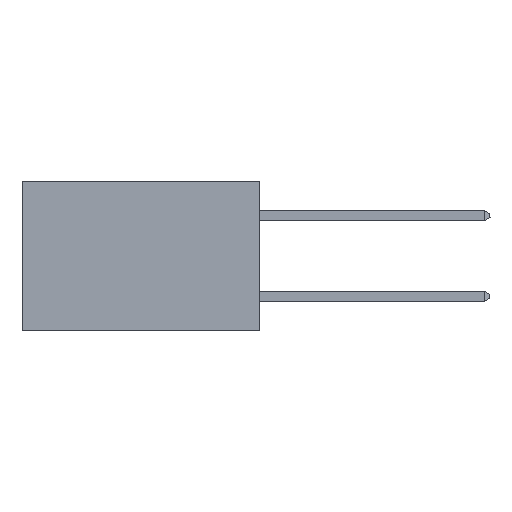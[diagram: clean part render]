
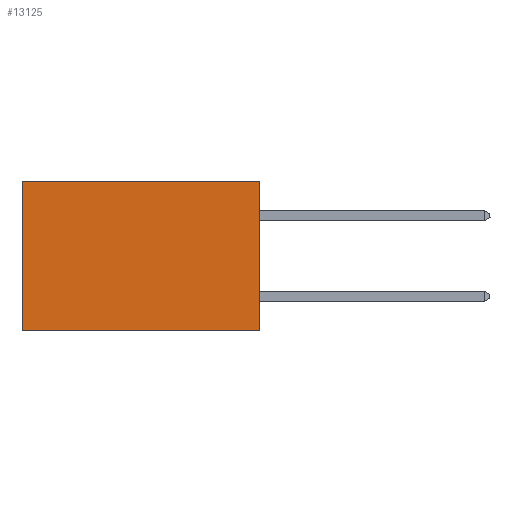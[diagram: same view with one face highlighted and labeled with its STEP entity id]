
A CAD part, left-side view. The second image highlights one B-rep face of the part: STEP entity #13125.
In plain terms, the highlighted planar face has unit normal (-1, 0, 0).
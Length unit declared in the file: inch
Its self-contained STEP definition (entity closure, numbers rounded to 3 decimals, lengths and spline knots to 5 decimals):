
#111 = VECTOR ( 'NONE', #22100, 39.37008 ) ;
#517 = VECTOR ( 'NONE', #2443, 39.37008 ) ;
#792 = CARTESIAN_POINT ( 'NONE',  ( 0.277, 0.59, -0.37 ) ) ;
#914 = CARTESIAN_POINT ( 'NONE',  ( 0.277, 0.59, -0.37 ) ) ;
#2443 = DIRECTION ( 'NONE',  ( 0., 0., -1. ) ) ;
#2617 = EDGE_CURVE ( 'NONE', #11484, #22022, #4882, .T. ) ;
#3557 = VECTOR ( 'NONE', #16718, 39.37008 ) ;
#4536 = LINE ( 'NONE', #6745, #22178 ) ;
#4661 = EDGE_CURVE ( 'NONE', #12851, #22022, #15409, .T. ) ;
#4882 = LINE ( 'NONE', #914, #517 ) ;
#5803 = CARTESIAN_POINT ( 'NONE',  ( 0.277, 0., -0.37 ) ) ;
#6662 = DIRECTION ( 'NONE',  ( 0., 1., 0. ) ) ;
#6679 = CARTESIAN_POINT ( 'NONE',  ( 0.277, 0., -0.37 ) ) ;
#6745 = CARTESIAN_POINT ( 'NONE',  ( 0.277, 0., 0. ) ) ;
#6975 = EDGE_CURVE ( 'NONE', #9878, #11484, #4536, .T. ) ;
#8498 = DIRECTION ( 'NONE',  ( 1., 0., 0. ) ) ;
#8901 = EDGE_CURVE ( 'NONE', #9878, #12851, #12826, .T. ) ;
#9401 = EDGE_LOOP ( 'NONE', ( #11407, #23289, #15206, #21095 ) ) ;
#9878 = VERTEX_POINT ( 'NONE', #19147 ) ;
#10684 = AXIS2_PLACEMENT_3D ( 'NONE', #6679, #8498, #21167 ) ;
#11407 = ORIENTED_EDGE ( 'NONE', *, *, #2617, .T. ) ;
#11484 = VERTEX_POINT ( 'NONE', #18402 ) ;
#12826 = LINE ( 'NONE', #5803, #3557 ) ;
#12851 = VERTEX_POINT ( 'NONE', #18588 ) ;
#13125 = ADVANCED_FACE ( 'NONE', ( #17720 ), #19385, .F. ) ;
#15206 = ORIENTED_EDGE ( 'NONE', *, *, #8901, .F. ) ;
#15409 = LINE ( 'NONE', #22102, #111 ) ;
#16718 = DIRECTION ( 'NONE',  ( 0., 0., -1. ) ) ;
#17720 = FACE_OUTER_BOUND ( 'NONE', #9401, .T. ) ;
#18402 = CARTESIAN_POINT ( 'NONE',  ( 0.277, 0.59, 0. ) ) ;
#18588 = CARTESIAN_POINT ( 'NONE',  ( 0.277, 0., -0.37 ) ) ;
#19147 = CARTESIAN_POINT ( 'NONE',  ( 0.277, 0., 0. ) ) ;
#19385 = PLANE ( 'NONE',  #10684 ) ;
#21095 = ORIENTED_EDGE ( 'NONE', *, *, #6975, .T. ) ;
#21167 = DIRECTION ( 'NONE',  ( 0., 0., -1. ) ) ;
#22022 = VERTEX_POINT ( 'NONE', #792 ) ;
#22100 = DIRECTION ( 'NONE',  ( 0., 1., 0. ) ) ;
#22102 = CARTESIAN_POINT ( 'NONE',  ( 0.277, 0., -0.37 ) ) ;
#22178 = VECTOR ( 'NONE', #6662, 39.37008 ) ;
#23289 = ORIENTED_EDGE ( 'NONE', *, *, #4661, .F. ) ;
